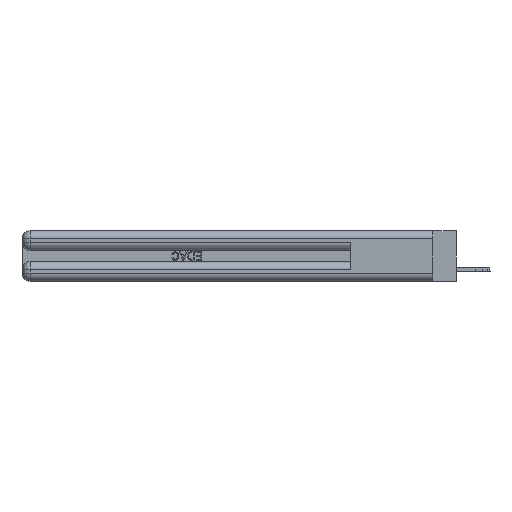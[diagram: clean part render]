
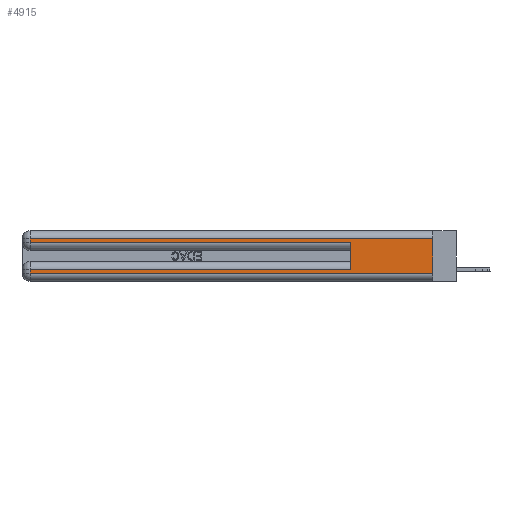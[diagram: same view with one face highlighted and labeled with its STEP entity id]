
A CAD part, left-side view. The second image highlights one B-rep face of the part: STEP entity #4915.
In plain terms, the highlighted planar face has unit normal (-1, 0, 0).
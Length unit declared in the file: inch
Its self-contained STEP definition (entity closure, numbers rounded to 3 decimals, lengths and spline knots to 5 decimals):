
#652 = ORIENTED_EDGE ( 'NONE', *, *, #10773, .T. ) ;
#826 = DIRECTION ( 'NONE',  ( 0., 1., 0. ) ) ;
#1516 = VECTOR ( 'NONE', #1589, 39.37008 ) ;
#1589 = DIRECTION ( 'NONE',  ( 0., 0., 1. ) ) ;
#1699 = LINE ( 'NONE', #2535, #23694 ) ;
#2370 = CARTESIAN_POINT ( 'NONE',  ( 0., 2.94, 0.285 ) ) ;
#2535 = CARTESIAN_POINT ( 'NONE',  ( 0., 2.94, 0.37 ) ) ;
#3695 = EDGE_CURVE ( 'NONE', #4105, #37607, #5577, .T. ) ;
#4105 = VERTEX_POINT ( 'NONE', #20131 ) ;
#4192 = DIRECTION ( 'NONE',  ( 0., 0., -1. ) ) ;
#4332 = ORIENTED_EDGE ( 'NONE', *, *, #39158, .F. ) ;
#4915 = ADVANCED_FACE ( 'NONE', ( #12735 ), #26073, .F. ) ;
#5003 = VECTOR ( 'NONE', #7772, 39.37008 ) ;
#5208 = CARTESIAN_POINT ( 'NONE',  ( 0., 2.94, 0.06 ) ) ;
#5557 = VERTEX_POINT ( 'NONE', #2370 ) ;
#5577 = LINE ( 'NONE', #11486, #10973 ) ;
#5611 = EDGE_CURVE ( 'NONE', #34556, #8777, #15172, .T. ) ;
#5673 = LINE ( 'NONE', #19220, #37983 ) ;
#6003 = VERTEX_POINT ( 'NONE', #10984 ) ;
#6859 = CARTESIAN_POINT ( 'NONE',  ( 0., 0., 0.31 ) ) ;
#7163 = DIRECTION ( 'NONE',  ( 1., 0., 0. ) ) ;
#7772 = DIRECTION ( 'NONE',  ( 0., 1., 0. ) ) ;
#8209 = AXIS2_PLACEMENT_3D ( 'NONE', #38822, #7163, #4192 ) ;
#8416 = CARTESIAN_POINT ( 'NONE',  ( 0., 0.6, 0.145 ) ) ;
#8777 = VERTEX_POINT ( 'NONE', #17595 ) ;
#9456 = CARTESIAN_POINT ( 'NONE',  ( 0., 2.94, 0.31 ) ) ;
#9959 = EDGE_CURVE ( 'NONE', #37607, #6003, #15976, .T. ) ;
#10773 = EDGE_CURVE ( 'NONE', #5557, #8777, #5673, .T. ) ;
#10973 = VECTOR ( 'NONE', #17815, 39.37008 ) ;
#10984 = CARTESIAN_POINT ( 'NONE',  ( 0., 0., 0.06 ) ) ;
#11474 = EDGE_CURVE ( 'NONE', #17468, #5557, #1699, .T. ) ;
#11486 = CARTESIAN_POINT ( 'NONE',  ( 0., 2.94, 0.37 ) ) ;
#11552 = EDGE_CURVE ( 'NONE', #39659, #17468, #26663, .T. ) ;
#12735 = FACE_OUTER_BOUND ( 'NONE', #21712, .T. ) ;
#15172 = LINE ( 'NONE', #8416, #1516 ) ;
#15610 = ORIENTED_EDGE ( 'NONE', *, *, #9959, .T. ) ;
#15617 = CARTESIAN_POINT ( 'NONE',  ( 0., 0., 0.31 ) ) ;
#15665 = DIRECTION ( 'NONE',  ( 0., 0., -1. ) ) ;
#15976 = LINE ( 'NONE', #22928, #37111 ) ;
#16300 = VECTOR ( 'NONE', #826, 39.37008 ) ;
#16990 = ORIENTED_EDGE ( 'NONE', *, *, #3695, .T. ) ;
#17151 = CARTESIAN_POINT ( 'NONE',  ( 0., 0.6, 0.085 ) ) ;
#17468 = VERTEX_POINT ( 'NONE', #9456 ) ;
#17595 = CARTESIAN_POINT ( 'NONE',  ( 0., 0.6, 0.285 ) ) ;
#17815 = DIRECTION ( 'NONE',  ( 0., 0., -1. ) ) ;
#19220 = CARTESIAN_POINT ( 'NONE',  ( 0., 0., 0.285 ) ) ;
#19669 = LINE ( 'NONE', #20244, #5003 ) ;
#20131 = CARTESIAN_POINT ( 'NONE',  ( 0., 2.94, 0.085 ) ) ;
#20244 = CARTESIAN_POINT ( 'NONE',  ( 0., 0., 0.085 ) ) ;
#20343 = ORIENTED_EDGE ( 'NONE', *, *, #11552, .T. ) ;
#21712 = EDGE_LOOP ( 'NONE', ( #4332, #20343, #21992, #652, #36132, #30369, #16990, #15610 ) ) ;
#21992 = ORIENTED_EDGE ( 'NONE', *, *, #11474, .T. ) ;
#22928 = CARTESIAN_POINT ( 'NONE',  ( 0., 0., 0.06 ) ) ;
#23694 = VECTOR ( 'NONE', #40164, 39.37008 ) ;
#25167 = DIRECTION ( 'NONE',  ( 0., -1., 0. ) ) ;
#25756 = LINE ( 'NONE', #34474, #35795 ) ;
#26073 = PLANE ( 'NONE',  #8209 ) ;
#26247 = DIRECTION ( 'NONE',  ( 0., -1., 0. ) ) ;
#26663 = LINE ( 'NONE', #6859, #16300 ) ;
#30369 = ORIENTED_EDGE ( 'NONE', *, *, #38155, .T. ) ;
#34474 = CARTESIAN_POINT ( 'NONE',  ( 0., 0., 0.37 ) ) ;
#34556 = VERTEX_POINT ( 'NONE', #17151 ) ;
#35795 = VECTOR ( 'NONE', #15665, 39.37008 ) ;
#36132 = ORIENTED_EDGE ( 'NONE', *, *, #5611, .F. ) ;
#37111 = VECTOR ( 'NONE', #26247, 39.37008 ) ;
#37607 = VERTEX_POINT ( 'NONE', #5208 ) ;
#37983 = VECTOR ( 'NONE', #25167, 39.37008 ) ;
#38155 = EDGE_CURVE ( 'NONE', #34556, #4105, #19669, .T. ) ;
#38822 = CARTESIAN_POINT ( 'NONE',  ( 0., 0., 0.37 ) ) ;
#39158 = EDGE_CURVE ( 'NONE', #39659, #6003, #25756, .T. ) ;
#39659 = VERTEX_POINT ( 'NONE', #15617 ) ;
#40164 = DIRECTION ( 'NONE',  ( 0., 0., -1. ) ) ;
